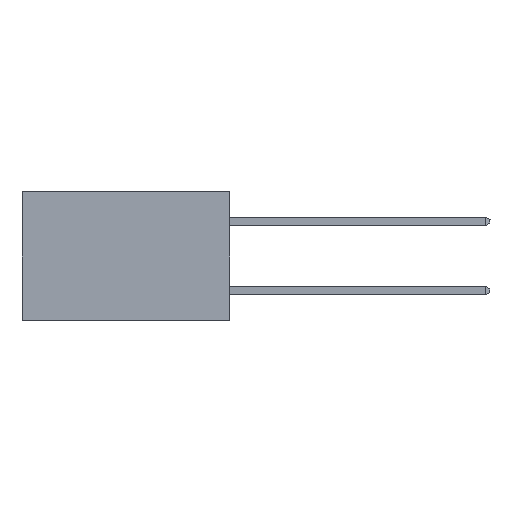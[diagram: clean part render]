
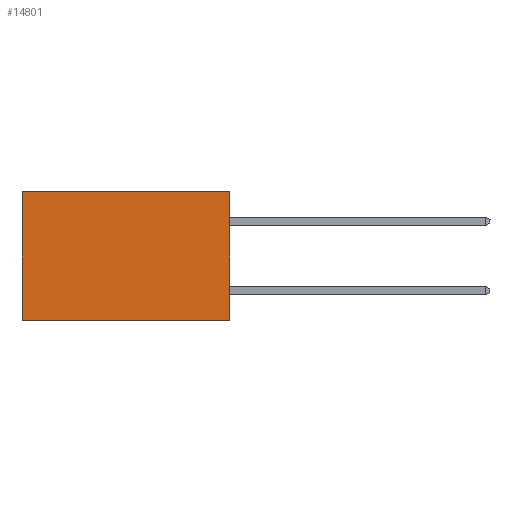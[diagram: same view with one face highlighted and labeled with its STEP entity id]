
A CAD part, left-side view. The second image highlights one B-rep face of the part: STEP entity #14801.
In plain terms, the highlighted planar face has unit normal (-1, 0, 0).
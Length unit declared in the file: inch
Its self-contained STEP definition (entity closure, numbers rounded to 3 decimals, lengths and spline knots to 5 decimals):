
#61 = VERTEX_POINT ( 'NONE', #6843 ) ;
#589 = EDGE_CURVE ( 'NONE', #13565, #6357, #4190, .T. ) ;
#926 = EDGE_CURVE ( 'NONE', #19232, #6357, #5397, .T. ) ;
#1444 = CARTESIAN_POINT ( 'NONE',  ( 0.2615, 0., -0.37 ) ) ;
#3551 = CARTESIAN_POINT ( 'NONE',  ( 0.2615, 0.6, -0.37 ) ) ;
#4190 = LINE ( 'NONE', #9829, #24142 ) ;
#4418 = DIRECTION ( 'NONE',  ( 0., 1., 0. ) ) ;
#5235 = DIRECTION ( 'NONE',  ( 1., 0., 0. ) ) ;
#5397 = LINE ( 'NONE', #3551, #6699 ) ;
#6089 = VECTOR ( 'NONE', #4418, 39.37008 ) ;
#6357 = VERTEX_POINT ( 'NONE', #7242 ) ;
#6676 = ORIENTED_EDGE ( 'NONE', *, *, #14668, .F. ) ;
#6699 = VECTOR ( 'NONE', #14332, 39.37008 ) ;
#6843 = CARTESIAN_POINT ( 'NONE',  ( 0.2615, 0., 0. ) ) ;
#7242 = CARTESIAN_POINT ( 'NONE',  ( 0.2615, 0.6, -0.37 ) ) ;
#8803 = DIRECTION ( 'NONE',  ( 0., 0., -1. ) ) ;
#9829 = CARTESIAN_POINT ( 'NONE',  ( 0.2615, 0., -0.37 ) ) ;
#10304 = CARTESIAN_POINT ( 'NONE',  ( 0.2615, 0., 0. ) ) ;
#10402 = CARTESIAN_POINT ( 'NONE',  ( 0.2615, 0., -0.37 ) ) ;
#10561 = EDGE_LOOP ( 'NONE', ( #17012, #17677, #6676, #24108 ) ) ;
#12698 = DIRECTION ( 'NONE',  ( 0., 0., -1. ) ) ;
#12933 = LINE ( 'NONE', #1444, #16675 ) ;
#12985 = EDGE_CURVE ( 'NONE', #61, #19232, #14084, .T. ) ;
#13358 = DIRECTION ( 'NONE',  ( 0., 1., 0. ) ) ;
#13565 = VERTEX_POINT ( 'NONE', #10402 ) ;
#14084 = LINE ( 'NONE', #10304, #6089 ) ;
#14332 = DIRECTION ( 'NONE',  ( 0., 0., -1. ) ) ;
#14668 = EDGE_CURVE ( 'NONE', #61, #13565, #12933, .T. ) ;
#14801 = ADVANCED_FACE ( 'NONE', ( #18079 ), #16249, .F. ) ;
#15300 = CARTESIAN_POINT ( 'NONE',  ( 0.2615, 0.6, 0. ) ) ;
#16249 = PLANE ( 'NONE',  #21775 ) ;
#16675 = VECTOR ( 'NONE', #8803, 39.37008 ) ;
#17012 = ORIENTED_EDGE ( 'NONE', *, *, #926, .T. ) ;
#17677 = ORIENTED_EDGE ( 'NONE', *, *, #589, .F. ) ;
#18079 = FACE_OUTER_BOUND ( 'NONE', #10561, .T. ) ;
#18330 = CARTESIAN_POINT ( 'NONE',  ( 0.2615, 0., -0.37 ) ) ;
#19232 = VERTEX_POINT ( 'NONE', #15300 ) ;
#21775 = AXIS2_PLACEMENT_3D ( 'NONE', #18330, #5235, #12698 ) ;
#24108 = ORIENTED_EDGE ( 'NONE', *, *, #12985, .T. ) ;
#24142 = VECTOR ( 'NONE', #13358, 39.37008 ) ;
